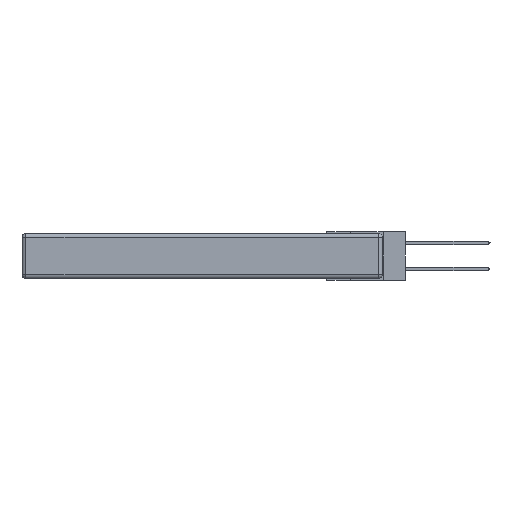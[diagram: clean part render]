
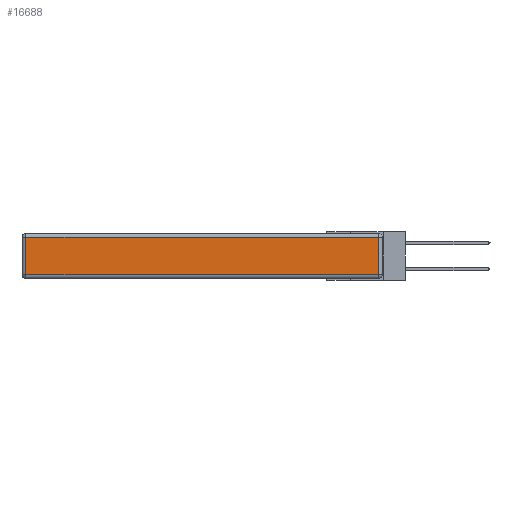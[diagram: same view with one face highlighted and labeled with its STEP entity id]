
A CAD part, left-side view. The second image highlights one B-rep face of the part: STEP entity #16688.
In plain terms, the highlighted planar face has unit normal (-1, 0, 0).
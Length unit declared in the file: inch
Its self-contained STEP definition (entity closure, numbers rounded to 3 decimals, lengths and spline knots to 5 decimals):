
#185 = DIRECTION ( 'NONE',  ( -1., 0., 0. ) ) ;
#269 = EDGE_CURVE ( 'NONE', #10178, #1245, #3093, .T. ) ;
#402 = CARTESIAN_POINT ( 'NONE',  ( 0., 0.03, -0.313 ) ) ;
#743 = EDGE_CURVE ( 'NONE', #16345, #5906, #11584, .T. ) ;
#1245 = VERTEX_POINT ( 'NONE', #402 ) ;
#1875 = AXIS2_PLACEMENT_3D ( 'NONE', #13093, #185, #9281 ) ;
#2375 = ORIENTED_EDGE ( 'NONE', *, *, #12553, .T. ) ;
#3093 = LINE ( 'NONE', #12296, #16439 ) ;
#4554 = DIRECTION ( 'NONE',  ( 0., -1., 0. ) ) ;
#5114 = VECTOR ( 'NONE', #11909, 39.37008 ) ;
#5555 = EDGE_LOOP ( 'NONE', ( #13265, #14519, #13129, #2375 ) ) ;
#5906 = VERTEX_POINT ( 'NONE', #9488 ) ;
#6677 = PLANE ( 'NONE',  #1875 ) ;
#7450 = CARTESIAN_POINT ( 'NONE',  ( 0., 0.03, -0.03 ) ) ;
#8043 = CARTESIAN_POINT ( 'NONE',  ( 0., 2.75, -0.03 ) ) ;
#8055 = CARTESIAN_POINT ( 'NONE',  ( 0., 2.72, -0.313 ) ) ;
#8409 = DIRECTION ( 'NONE',  ( 0., 0., 1. ) ) ;
#9281 = DIRECTION ( 'NONE',  ( 0., 0., 1. ) ) ;
#9488 = CARTESIAN_POINT ( 'NONE',  ( 0., 2.72, -0.03 ) ) ;
#9663 = LINE ( 'NONE', #11344, #11242 ) ;
#10178 = VERTEX_POINT ( 'NONE', #8055 ) ;
#10367 = DIRECTION ( 'NONE',  ( 0., 0., -1. ) ) ;
#10865 = VECTOR ( 'NONE', #8409, 39.37008 ) ;
#11242 = VECTOR ( 'NONE', #10367, 39.37008 ) ;
#11344 = CARTESIAN_POINT ( 'NONE',  ( 0., 2.72, -0.343 ) ) ;
#11367 = FACE_OUTER_BOUND ( 'NONE', #5555, .T. ) ;
#11584 = LINE ( 'NONE', #8043, #5114 ) ;
#11909 = DIRECTION ( 'NONE',  ( 0., 1., 0. ) ) ;
#12296 = CARTESIAN_POINT ( 'NONE',  ( 0., 0., -0.313 ) ) ;
#12553 = EDGE_CURVE ( 'NONE', #5906, #10178, #9663, .T. ) ;
#12656 = LINE ( 'NONE', #14800, #10865 ) ;
#13093 = CARTESIAN_POINT ( 'NONE',  ( 0., 0., -0.343 ) ) ;
#13129 = ORIENTED_EDGE ( 'NONE', *, *, #743, .T. ) ;
#13265 = ORIENTED_EDGE ( 'NONE', *, *, #269, .T. ) ;
#14519 = ORIENTED_EDGE ( 'NONE', *, *, #14672, .T. ) ;
#14672 = EDGE_CURVE ( 'NONE', #1245, #16345, #12656, .T. ) ;
#14800 = CARTESIAN_POINT ( 'NONE',  ( 0., 0.03, -0.343 ) ) ;
#16345 = VERTEX_POINT ( 'NONE', #7450 ) ;
#16439 = VECTOR ( 'NONE', #4554, 39.37008 ) ;
#16688 = ADVANCED_FACE ( 'NONE', ( #11367 ), #6677, .T. ) ;
